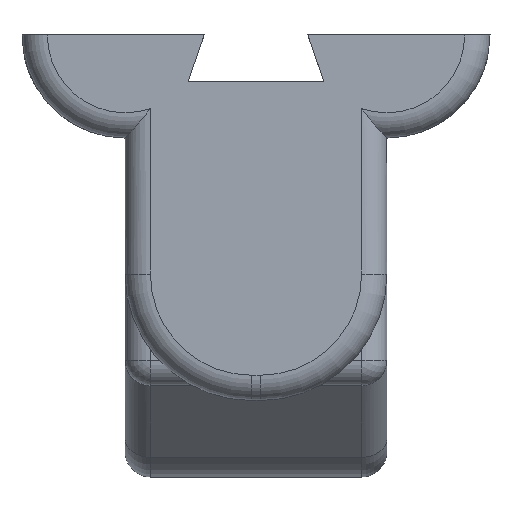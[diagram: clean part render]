
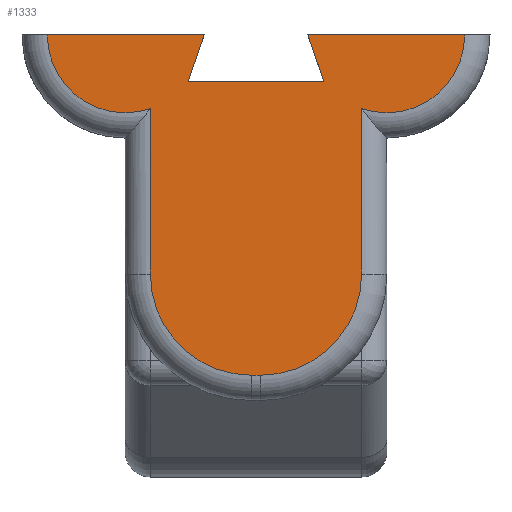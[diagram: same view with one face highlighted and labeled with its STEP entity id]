
A CAD part, front view. The second image highlights one B-rep face of the part: STEP entity #1333.
In plain terms, the highlighted planar face has unit normal (0, -1, 0).
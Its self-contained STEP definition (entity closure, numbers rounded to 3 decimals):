
#62=LINE('',#2092,#158);
#66=LINE('',#2100,#162);
#67=LINE('',#2104,#163);
#68=LINE('',#2108,#164);
#69=LINE('',#2112,#165);
#70=LINE('',#2114,#166);
#71=LINE('',#2116,#167);
#72=LINE('',#2117,#168);
#158=VECTOR('',#1621,10.);
#162=VECTOR('',#1627,10.);
#163=VECTOR('',#1630,10.);
#164=VECTOR('',#1633,10.);
#165=VECTOR('',#1636,10.);
#166=VECTOR('',#1637,10.);
#167=VECTOR('',#1638,10.);
#168=VECTOR('',#1639,10.);
#255=PLANE('',#1434);
#279=FACE_OUTER_BOUND('',#363,.T.);
#363=EDGE_LOOP('',(#896,#897,#898,#899,#900,#901,#902,#903,#904,#905,#906,
#907));
#467=CIRCLE('',#1432,6.15);
#468=CIRCLE('',#1435,8.);
#469=CIRCLE('',#1436,8.);
#470=CIRCLE('',#1437,6.15);
#553=VERTEX_POINT('',#2069);
#556=VERTEX_POINT('',#2074);
#557=VERTEX_POINT('',#2091);
#560=VERTEX_POINT('',#2099);
#561=VERTEX_POINT('',#2101);
#562=VERTEX_POINT('',#2103);
#563=VERTEX_POINT('',#2105);
#564=VERTEX_POINT('',#2107);
#565=VERTEX_POINT('',#2109);
#566=VERTEX_POINT('',#2111);
#567=VERTEX_POINT('',#2113);
#568=VERTEX_POINT('',#2115);
#680=EDGE_CURVE('',#556,#553,#467,.T.);
#681=EDGE_CURVE('',#553,#557,#62,.T.);
#685=EDGE_CURVE('',#560,#556,#66,.T.);
#686=EDGE_CURVE('',#561,#560,#468,.T.);
#687=EDGE_CURVE('',#562,#561,#67,.T.);
#688=EDGE_CURVE('',#563,#562,#469,.T.);
#689=EDGE_CURVE('',#564,#563,#68,.T.);
#690=EDGE_CURVE('',#565,#564,#470,.T.);
#691=EDGE_CURVE('',#566,#565,#69,.T.);
#692=EDGE_CURVE('',#566,#567,#70,.T.);
#693=EDGE_CURVE('',#567,#568,#71,.T.);
#694=EDGE_CURVE('',#568,#557,#72,.T.);
#896=ORIENTED_EDGE('',*,*,#680,.F.);
#897=ORIENTED_EDGE('',*,*,#685,.F.);
#898=ORIENTED_EDGE('',*,*,#686,.F.);
#899=ORIENTED_EDGE('',*,*,#687,.F.);
#900=ORIENTED_EDGE('',*,*,#688,.F.);
#901=ORIENTED_EDGE('',*,*,#689,.F.);
#902=ORIENTED_EDGE('',*,*,#690,.F.);
#903=ORIENTED_EDGE('',*,*,#691,.F.);
#904=ORIENTED_EDGE('',*,*,#692,.T.);
#905=ORIENTED_EDGE('',*,*,#693,.T.);
#906=ORIENTED_EDGE('',*,*,#694,.T.);
#907=ORIENTED_EDGE('',*,*,#681,.F.);
#1333=ADVANCED_FACE('',(#279),#255,.F.);
#1432=AXIS2_PLACEMENT_3D('',#2089,#1617,#1618);
#1434=AXIS2_PLACEMENT_3D('',#2098,#1625,#1626);
#1435=AXIS2_PLACEMENT_3D('',#2102,#1628,#1629);
#1436=AXIS2_PLACEMENT_3D('',#2106,#1631,#1632);
#1437=AXIS2_PLACEMENT_3D('',#2110,#1634,#1635);
#1617=DIRECTION('center_axis',(0.,1.,0.));
#1618=DIRECTION('ref_axis',(-0.614,0.,-0.789));
#1621=DIRECTION('',(1.,0.,0.));
#1625=DIRECTION('center_axis',(0.,1.,0.));
#1626=DIRECTION('ref_axis',(1.,0.,0.));
#1627=DIRECTION('',(0.,0.,1.));
#1628=DIRECTION('center_axis',(0.,1.,0.));
#1629=DIRECTION('ref_axis',(-0.707,0.,-0.707));
#1630=DIRECTION('',(-1.,0.,0.));
#1631=DIRECTION('center_axis',(0.,1.,0.));
#1632=DIRECTION('ref_axis',(0.707,0.,-0.707));
#1633=DIRECTION('',(0.,0.,-1.));
#1634=DIRECTION('center_axis',(0.,1.,0.));
#1635=DIRECTION('ref_axis',(0.614,0.,-0.789));
#1636=DIRECTION('',(1.,0.,0.));
#1637=DIRECTION('',(0.328,0.,-0.945));
#1638=DIRECTION('',(-1.,0.,0.));
#1639=DIRECTION('',(0.328,0.,0.945));
#2069=CARTESIAN_POINT('',(2.,0.,8.15));
#2074=CARTESIAN_POINT('',(10.15,0.,2.334));
#2089=CARTESIAN_POINT('Origin',(8.15,0.,8.15));
#2091=CARTESIAN_POINT('',(14.4,0.,8.15));
#2092=CARTESIAN_POINT('',(0.,0.,8.15));
#2098=CARTESIAN_POINT('Origin',(18.5,0.,4.075));
#2099=CARTESIAN_POINT('',(10.15,0.,-10.75));
#2100=CARTESIAN_POINT('',(10.15,0.,-3.15));
#2101=CARTESIAN_POINT('',(18.15,0.,-18.75));
#2102=CARTESIAN_POINT('Origin',(18.15,0.,-10.75));
#2103=CARTESIAN_POINT('',(18.85,0.,-18.75));
#2104=CARTESIAN_POINT('',(18.5,0.,-18.75));
#2105=CARTESIAN_POINT('',(26.85,0.,-10.75));
#2106=CARTESIAN_POINT('Origin',(18.85,0.,-10.75));
#2107=CARTESIAN_POINT('',(26.85,0.,2.334));
#2108=CARTESIAN_POINT('',(26.85,0.,-3.15));
#2109=CARTESIAN_POINT('',(35.,0.,8.15));
#2110=CARTESIAN_POINT('Origin',(28.85,0.,8.15));
#2111=CARTESIAN_POINT('',(22.6,0.,8.15));
#2112=CARTESIAN_POINT('',(0.,0.,8.15));
#2113=CARTESIAN_POINT('',(23.875,0.,4.48));
#2114=CARTESIAN_POINT('',(23.011,0.,6.967));
#2115=CARTESIAN_POINT('',(13.125,0.,4.48));
#2116=CARTESIAN_POINT('',(21.188,0.,4.48));
#2117=CARTESIAN_POINT('',(13.352,0.,5.132));
